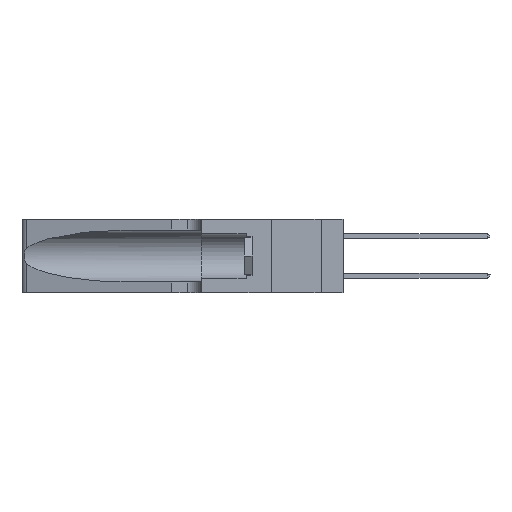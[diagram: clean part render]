
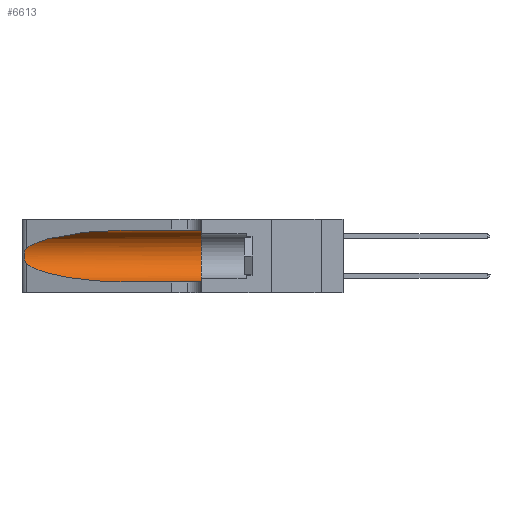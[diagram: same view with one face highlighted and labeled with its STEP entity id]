
A CAD part, left-side view. The second image highlights one B-rep face of the part: STEP entity #6613.
In plain terms, the highlighted cylindrical face has radius 3.308 mm (diameter 6.617 mm), a partial arc.
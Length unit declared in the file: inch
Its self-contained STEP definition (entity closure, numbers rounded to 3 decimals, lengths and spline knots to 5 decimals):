
#93 = LINE ( 'NONE', #15217, #17778 ) ;
#95 = CARTESIAN_POINT ( 'NONE',  ( 0.25639, 1.23186, 0.15144 ) ) ;
#190 = CARTESIAN_POINT ( 'NONE',  ( 0.25854, 1.2359, 0.20912 ) ) ;
#891 = EDGE_CURVE ( 'NONE', #18533, #18869, #6566, .T. ) ;
#952 = EDGE_CURVE ( 'NONE', #25009, #18533, #23300, .T. ) ;
#964 = CARTESIAN_POINT ( 'NONE',  ( 0.1305, 0.72297, 0.05475 ) ) ;
#2026 = CARTESIAN_POINT ( 'NONE',  ( 0.25487, 1.22718, 0.22369 ) ) ;
#2113 = AXIS2_PLACEMENT_3D ( 'NONE', #5975, #18113, #3783 ) ;
#2115 = CARTESIAN_POINT ( 'NONE',  ( 0.26075, 1.23896, 0.178 ) ) ;
#2538 = DIRECTION ( 'NONE',  ( 0., 0., -1. ) ) ;
#2719 = CARTESIAN_POINT ( 'NONE',  ( 0.1305, 1.61858, 0.185 ) ) ;
#2857 = EDGE_LOOP ( 'NONE', ( #22982, #9832, #23472, #4361, #8903, #8565 ) ) ;
#3108 = VECTOR ( 'NONE', #10763, 39.37008 ) ;
#3547 = VERTEX_POINT ( 'NONE', #12179 ) ;
#3783 = DIRECTION ( 'NONE',  ( 0., 0., 1. ) ) ;
#4059 = CARTESIAN_POINT ( 'NONE',  ( 0.26017, 1.23833, 0.17102 ) ) ;
#4136 = CARTESIAN_POINT ( 'NONE',  ( 0.2373, 1.15595, 0.28018 ) ) ;
#4149 = CARTESIAN_POINT ( 'NONE',  ( 0.25639, 1.23184, 0.21858 ) ) ;
#4313 = CARTESIAN_POINT ( 'NONE',  ( 0.1305, 0.72297, 0.31525 ) ) ;
#4361 = ORIENTED_EDGE ( 'NONE', *, *, #891, .T. ) ;
#4480 = VERTEX_POINT ( 'NONE', #14967 ) ;
#5624 = CARTESIAN_POINT ( 'NONE',  ( 0.25487, 1.22718, 0.14631 ) ) ;
#5975 = CARTESIAN_POINT ( 'NONE',  ( 0.1305, 0.35, 0.185 ) ) ;
#6516 = CARTESIAN_POINT ( 'NONE',  ( 0.1305, 1.61858, 0.05475 ) ) ;
#6566 = LINE ( 'NONE', #6516, #3108 ) ;
#6613 = ADVANCED_FACE ( 'NONE', ( #18603 ), #25538, .F. ) ;
#6763 = CIRCLE ( 'NONE', #2113, 0.13025 ) ;
#8565 = ORIENTED_EDGE ( 'NONE', *, *, #14243, .F. ) ;
#8737 = EDGE_CURVE ( 'NONE', #3547, #4480, #15004, .T. ) ;
#8903 = ORIENTED_EDGE ( 'NONE', *, *, #23076, .F. ) ;
#9832 = ORIENTED_EDGE ( 'NONE', *, *, #19929, .T. ) ;
#10077 = CARTESIAN_POINT ( 'NONE',  ( 0.1305, 0.72297, 0.05475 ) ) ;
#10343 = CARTESIAN_POINT ( 'NONE',  ( 0.25555, 1.22993, 0.14849 ) ) ;
#10763 = DIRECTION ( 'NONE',  ( 0., -1., 0. ) ) ;
#12164 = CARTESIAN_POINT ( 'NONE',  ( 0.25856, 1.23593, 0.16098 ) ) ;
#12179 = CARTESIAN_POINT ( 'NONE',  ( 0.1305, 0.72297, 0.31525 ) ) ;
#12402 = CARTESIAN_POINT ( 'NONE',  ( 0.25487, 1.22718, 0.22369 ) ) ;
#12942 = CARTESIAN_POINT ( 'NONE',  ( 0.18966, 0.96281, 0.05475 ) ) ;
#13115 = CARTESIAN_POINT ( 'NONE',  ( 0.25487, 1.22718, 0.14631 ) ) ;
#14243 = EDGE_CURVE ( 'NONE', #3547, #24688, #93, .T. ) ;
#14380 = CARTESIAN_POINT ( 'NONE',  ( 0.25789, 1.23486, 0.15765 ) ) ;
#14967 = CARTESIAN_POINT ( 'NONE',  ( 0.25487, 1.22718, 0.22369 ) ) ;
#15001 = CARTESIAN_POINT ( 'NONE',  ( 0.1305, 0.35, 0.31525 ) ) ;
#15004 =( BOUNDED_CURVE ( )  B_SPLINE_CURVE ( 3, ( #4313, #18482, #4136, #12402 ),
 .UNSPECIFIED., .F., .F. ) 
 B_SPLINE_CURVE_WITH_KNOTS ( ( 4, 4 ),
 ( 1.5708, 2.84003 ),
 .UNSPECIFIED. ) 
 CURVE ( )  GEOMETRIC_REPRESENTATION_ITEM ( )  RATIONAL_B_SPLINE_CURVE ( ( 1., 0.87, 0.87, 1. ) ) 
 REPRESENTATION_ITEM ( '' )  );
#15217 = CARTESIAN_POINT ( 'NONE',  ( 0.1305, 1.61858, 0.31525 ) ) ;
#15982 = CARTESIAN_POINT ( 'NONE',  ( 0.1305, 0.35, 0.05475 ) ) ;
#16189 = CARTESIAN_POINT ( 'NONE',  ( 0.25787, 1.23484, 0.2124 ) ) ;
#17778 = VECTOR ( 'NONE', #21273, 39.37008 ) ;
#18113 = DIRECTION ( 'NONE',  ( 0., 1., 0. ) ) ;
#18440 = AXIS2_PLACEMENT_3D ( 'NONE', #2719, #24999, #2538 ) ;
#18482 = CARTESIAN_POINT ( 'NONE',  ( 0.18966, 0.96281, 0.31525 ) ) ;
#18533 = VERTEX_POINT ( 'NONE', #10077 ) ;
#18603 = FACE_OUTER_BOUND ( 'NONE', #2857, .T. ) ;
#18869 = VERTEX_POINT ( 'NONE', #15982 ) ;
#19929 = EDGE_CURVE ( 'NONE', #4480, #25009, #20872, .T. ) ;
#20431 = CARTESIAN_POINT ( 'NONE',  ( 0.25555, 1.22994, 0.2215 ) ) ;
#20872 = B_SPLINE_CURVE_WITH_KNOTS ( 'NONE', 3,
 ( #2026, #20431, #4149, #16189, #190, #24669, #24411, #2115, #4059, #12164, #14380, #95, #10343, #22541 ),
 .UNSPECIFIED., .F., .F.,
 ( 4, 2, 2, 2, 2, 2, 4 ),
 ( 0., 0.00027, 0.00053, 0.00107, 0.0016, 0.00187, 0.00214 ),
 .UNSPECIFIED. ) ;
#20944 = CARTESIAN_POINT ( 'NONE',  ( 0.2373, 1.15595, 0.08982 ) ) ;
#21273 = DIRECTION ( 'NONE',  ( 0., -1., 0. ) ) ;
#22541 = CARTESIAN_POINT ( 'NONE',  ( 0.25487, 1.22718, 0.14631 ) ) ;
#22982 = ORIENTED_EDGE ( 'NONE', *, *, #8737, .T. ) ;
#23076 = EDGE_CURVE ( 'NONE', #24688, #18869, #6763, .T. ) ;
#23300 =( BOUNDED_CURVE ( )  B_SPLINE_CURVE ( 3, ( #13115, #20944, #12942, #964 ),
 .UNSPECIFIED., .F., .F. ) 
 B_SPLINE_CURVE_WITH_KNOTS ( ( 4, 4 ),
 ( 3.44316, 4.71239 ),
 .UNSPECIFIED. ) 
 CURVE ( )  GEOMETRIC_REPRESENTATION_ITEM ( )  RATIONAL_B_SPLINE_CURVE ( ( 1., 0.87, 0.87, 1. ) ) 
 REPRESENTATION_ITEM ( '' )  );
#23472 = ORIENTED_EDGE ( 'NONE', *, *, #952, .T. ) ;
#24411 = CARTESIAN_POINT ( 'NONE',  ( 0.26075, 1.23896, 0.19203 ) ) ;
#24669 = CARTESIAN_POINT ( 'NONE',  ( 0.26018, 1.23835, 0.19895 ) ) ;
#24688 = VERTEX_POINT ( 'NONE', #15001 ) ;
#24999 = DIRECTION ( 'NONE',  ( 0., -1., 0. ) ) ;
#25009 = VERTEX_POINT ( 'NONE', #5624 ) ;
#25538 = CYLINDRICAL_SURFACE ( 'NONE', #18440, 0.13025 ) ;
